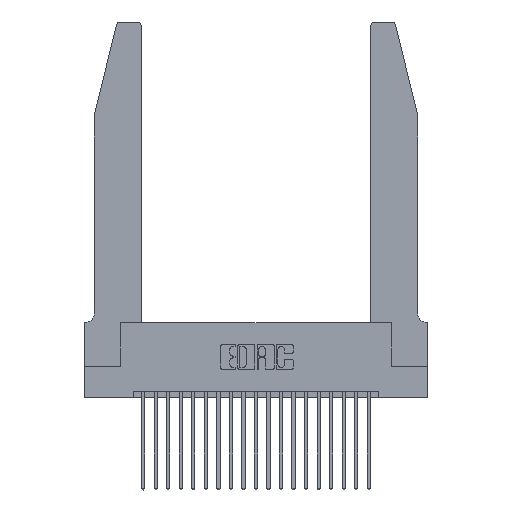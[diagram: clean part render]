
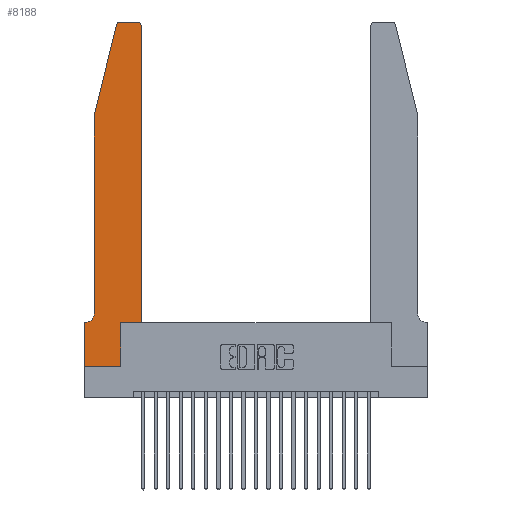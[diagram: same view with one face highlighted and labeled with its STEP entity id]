
A CAD part, top view. The second image highlights one B-rep face of the part: STEP entity #8188.
In plain terms, the highlighted planar face has unit normal (0, 0, 1).
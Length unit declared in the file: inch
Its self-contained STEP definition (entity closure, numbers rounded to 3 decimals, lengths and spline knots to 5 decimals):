
#153 = CARTESIAN_POINT ( 'NONE',  ( 0.0755, 0.35, 0.37 ) ) ;
#499 = DIRECTION ( 'NONE',  ( 0., 0., -1. ) ) ;
#976 = DIRECTION ( 'NONE',  ( 0., 0., 1. ) ) ;
#1035 = LINE ( 'NONE', #20584, #7423 ) ;
#1131 = EDGE_CURVE ( 'NONE', #19351, #13628, #3426, .T. ) ;
#1167 = VERTEX_POINT ( 'NONE', #3401 ) ;
#1237 = VERTEX_POINT ( 'NONE', #10585 ) ;
#1356 = CARTESIAN_POINT ( 'NONE',  ( 0., 0.35, 0.37 ) ) ;
#1400 = CARTESIAN_POINT ( 'NONE',  ( 0., 0., 0.37 ) ) ;
#1455 = EDGE_CURVE ( 'NONE', #13628, #8758, #8399, .T. ) ;
#2213 = DIRECTION ( 'NONE',  ( -1., 0., 0. ) ) ;
#2496 = CARTESIAN_POINT ( 'NONE',  ( 0.0055, 0.42, 0.37 ) ) ;
#2567 = DIRECTION ( 'NONE',  ( 1., 0., 0. ) ) ;
#2733 = DIRECTION ( 'NONE',  ( 1., 0., 0. ) ) ;
#3032 = DIRECTION ( 'NONE',  ( 0., -1., 0. ) ) ;
#3401 = CARTESIAN_POINT ( 'NONE',  ( 0.4505, 0.35, 0.37 ) ) ;
#3426 = LINE ( 'NONE', #153, #19651 ) ;
#3820 = CARTESIAN_POINT ( 'NONE',  ( 0.0755, 2., 0.37 ) ) ;
#4008 = AXIS2_PLACEMENT_3D ( 'NONE', #14590, #11225, #9616 ) ;
#4113 = EDGE_CURVE ( 'NONE', #4849, #8094, #4987, .T. ) ;
#4429 = EDGE_CURVE ( 'NONE', #1237, #14516, #5264, .T. ) ;
#4613 = CARTESIAN_POINT ( 'NONE',  ( 0.4205, 2.72, 0.37 ) ) ;
#4625 = EDGE_CURVE ( 'NONE', #8094, #19529, #7200, .T. ) ;
#4849 = VERTEX_POINT ( 'NONE', #7560 ) ;
#4987 = LINE ( 'NONE', #3820, #6937 ) ;
#5264 = CIRCLE ( 'NONE', #18877, 0.03 ) ;
#5388 = ORIENTED_EDGE ( 'NONE', *, *, #10238, .T. ) ;
#5432 = DIRECTION ( 'NONE',  ( 0., -1., 0. ) ) ;
#5707 = DIRECTION ( 'NONE',  ( -1., 0., 0. ) ) ;
#5842 = ORIENTED_EDGE ( 'NONE', *, *, #15284, .T. ) ;
#6172 = CARTESIAN_POINT ( 'NONE',  ( 0.0055, 0.35, 0.37 ) ) ;
#6601 = CARTESIAN_POINT ( 'NONE',  ( 0., 0., 0.37 ) ) ;
#6773 = AXIS2_PLACEMENT_3D ( 'NONE', #15613, #11954, #15376 ) ;
#6937 = VECTOR ( 'NONE', #21335, 39.37008 ) ;
#7050 = LINE ( 'NONE', #21705, #17183 ) ;
#7200 = LINE ( 'NONE', #7370, #11028 ) ;
#7281 = EDGE_CURVE ( 'NONE', #19529, #19351, #10219, .T. ) ;
#7370 = CARTESIAN_POINT ( 'NONE',  ( 0.0755, 2., 0.37 ) ) ;
#7423 = VECTOR ( 'NONE', #13638, 39.37008 ) ;
#7560 = CARTESIAN_POINT ( 'NONE',  ( 0.25487, 2.72718, 0.37 ) ) ;
#7633 = VECTOR ( 'NONE', #5707, 39.37008 ) ;
#8094 = VERTEX_POINT ( 'NONE', #20714 ) ;
#8188 = ADVANCED_FACE ( 'NONE', ( #10690 ), #21174, .T. ) ;
#8399 = LINE ( 'NONE', #1400, #18289 ) ;
#8469 = EDGE_CURVE ( 'NONE', #14516, #19959, #9302, .T. ) ;
#8728 = VECTOR ( 'NONE', #21862, 39.37008 ) ;
#8758 = VERTEX_POINT ( 'NONE', #6601 ) ;
#9228 = CARTESIAN_POINT ( 'NONE',  ( 0.4205, 2.75, 0.37 ) ) ;
#9302 = LINE ( 'NONE', #16505, #7633 ) ;
#9390 = CARTESIAN_POINT ( 'NONE',  ( 0.4505, 0.35, 0.37 ) ) ;
#9616 = DIRECTION ( 'NONE',  ( 1., 0., 0. ) ) ;
#10203 = AXIS2_PLACEMENT_3D ( 'NONE', #2496, #499, #2213 ) ;
#10219 = CIRCLE ( 'NONE', #10203, 0.07 ) ;
#10238 = EDGE_CURVE ( 'NONE', #1167, #1237, #7050, .T. ) ;
#10304 = ORIENTED_EDGE ( 'NONE', *, *, #22389, .T. ) ;
#10585 = CARTESIAN_POINT ( 'NONE',  ( 0.4505, 2.72, 0.37 ) ) ;
#10690 = FACE_OUTER_BOUND ( 'NONE', #14043, .T. ) ;
#10768 = ORIENTED_EDGE ( 'NONE', *, *, #1455, .T. ) ;
#11028 = VECTOR ( 'NONE', #5432, 39.37008 ) ;
#11062 = DIRECTION ( 'NONE',  ( 0., 1., 0. ) ) ;
#11225 = DIRECTION ( 'NONE',  ( 0., 0., 1. ) ) ;
#11954 = DIRECTION ( 'NONE',  ( 0., 0., 1. ) ) ;
#12000 = CARTESIAN_POINT ( 'NONE',  ( 0.0755, 0.42, 0.37 ) ) ;
#12579 = ORIENTED_EDGE ( 'NONE', *, *, #8469, .T. ) ;
#13489 = CIRCLE ( 'NONE', #6773, 0.03 ) ;
#13593 = EDGE_CURVE ( 'NONE', #19959, #4849, #13489, .T. ) ;
#13628 = VERTEX_POINT ( 'NONE', #1356 ) ;
#13638 = DIRECTION ( 'NONE',  ( 0., 1., 0. ) ) ;
#13797 = CARTESIAN_POINT ( 'NONE',  ( 0.2865, 0.35, 0.37 ) ) ;
#14043 = EDGE_LOOP ( 'NONE', ( #12579, #14426, #17366, #19976, #15444, #21533, #10768, #21665, #5842, #10304, #5388, #15282 ) ) ;
#14218 = LINE ( 'NONE', #9390, #8728 ) ;
#14426 = ORIENTED_EDGE ( 'NONE', *, *, #13593, .T. ) ;
#14516 = VERTEX_POINT ( 'NONE', #9228 ) ;
#14590 = CARTESIAN_POINT ( 'NONE',  ( 0., 0.35, 0.37 ) ) ;
#14823 = VERTEX_POINT ( 'NONE', #13797 ) ;
#15282 = ORIENTED_EDGE ( 'NONE', *, *, #4429, .T. ) ;
#15284 = EDGE_CURVE ( 'NONE', #18168, #14823, #1035, .T. ) ;
#15376 = DIRECTION ( 'NONE',  ( 1., 0., 0. ) ) ;
#15444 = ORIENTED_EDGE ( 'NONE', *, *, #7281, .T. ) ;
#15613 = CARTESIAN_POINT ( 'NONE',  ( 0.284, 2.72, 0.37 ) ) ;
#15720 = DIRECTION ( 'NONE',  ( -1., 0., 0. ) ) ;
#16354 = CARTESIAN_POINT ( 'NONE',  ( 0., 0., 0.37 ) ) ;
#16505 = CARTESIAN_POINT ( 'NONE',  ( 0.2605, 2.75, 0.37 ) ) ;
#17183 = VECTOR ( 'NONE', #11062, 39.37008 ) ;
#17366 = ORIENTED_EDGE ( 'NONE', *, *, #4113, .T. ) ;
#18070 = VECTOR ( 'NONE', #2567, 39.37008 ) ;
#18168 = VERTEX_POINT ( 'NONE', #19725 ) ;
#18289 = VECTOR ( 'NONE', #3032, 39.37008 ) ;
#18877 = AXIS2_PLACEMENT_3D ( 'NONE', #4613, #976, #2733 ) ;
#19351 = VERTEX_POINT ( 'NONE', #6172 ) ;
#19529 = VERTEX_POINT ( 'NONE', #12000 ) ;
#19651 = VECTOR ( 'NONE', #15720, 39.37008 ) ;
#19725 = CARTESIAN_POINT ( 'NONE',  ( 0.2865, 0., 0.37 ) ) ;
#19959 = VERTEX_POINT ( 'NONE', #22068 ) ;
#19976 = ORIENTED_EDGE ( 'NONE', *, *, #4625, .T. ) ;
#20584 = CARTESIAN_POINT ( 'NONE',  ( 0.2865, 0.35, 0.37 ) ) ;
#20714 = CARTESIAN_POINT ( 'NONE',  ( 0.0755, 2., 0.37 ) ) ;
#21174 = PLANE ( 'NONE',  #4008 ) ;
#21335 = DIRECTION ( 'NONE',  ( -0.239, -0.971, 0. ) ) ;
#21533 = ORIENTED_EDGE ( 'NONE', *, *, #1131, .T. ) ;
#21665 = ORIENTED_EDGE ( 'NONE', *, *, #22362, .T. ) ;
#21705 = CARTESIAN_POINT ( 'NONE',  ( 0.4505, 0.35, 0.37 ) ) ;
#21862 = DIRECTION ( 'NONE',  ( 1., 0., 0. ) ) ;
#22068 = CARTESIAN_POINT ( 'NONE',  ( 0.284, 2.75, 0.37 ) ) ;
#22362 = EDGE_CURVE ( 'NONE', #8758, #18168, #22711, .T. ) ;
#22389 = EDGE_CURVE ( 'NONE', #14823, #1167, #14218, .T. ) ;
#22711 = LINE ( 'NONE', #16354, #18070 ) ;
